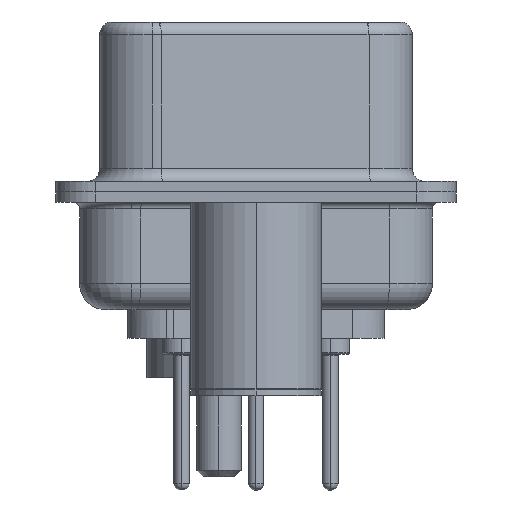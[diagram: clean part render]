
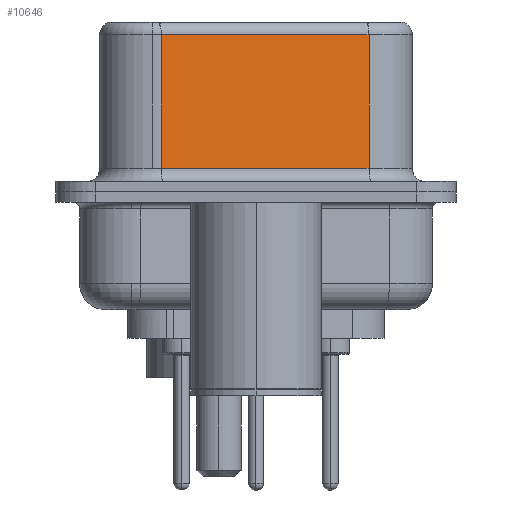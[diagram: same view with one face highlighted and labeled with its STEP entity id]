
A CAD part, left-side view. The second image highlights one B-rep face of the part: STEP entity #10646.
In plain terms, the highlighted planar face has unit normal (-0.985, -0.174, 0).
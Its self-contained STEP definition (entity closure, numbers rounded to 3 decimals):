
#1624 = CARTESIAN_POINT ( 'NONE',  ( 5.132, -4.322, 6.52 ) ) ;
#1778 = DIRECTION ( 'NONE',  ( 0., 0., -1. ) ) ;
#2152 = FACE_OUTER_BOUND ( 'NONE', #5448, .T. ) ;
#3857 = EDGE_CURVE ( 'NONE', #17078, #5729, #20822, .T. ) ;
#3877 = DIRECTION ( 'NONE',  ( -0.174, 0.985, 0. ) ) ;
#4196 = EDGE_CURVE ( 'NONE', #9244, #5729, #7252, .T. ) ;
#4510 = CARTESIAN_POINT ( 'NONE',  ( 5.132, -4.322, 6.52 ) ) ;
#4956 = VECTOR ( 'NONE', #6572, 1000. ) ;
#5448 = EDGE_LOOP ( 'NONE', ( #12501, #22151, #11166, #16965 ) ) ;
#5729 = VERTEX_POINT ( 'NONE', #16678 ) ;
#6572 = DIRECTION ( 'NONE',  ( 0., 0., -1. ) ) ;
#6870 = CARTESIAN_POINT ( 'NONE',  ( 5.132, -4.322, 6.02 ) ) ;
#7252 = LINE ( 'NONE', #4510, #12563 ) ;
#7342 = EDGE_CURVE ( 'NONE', #9244, #25363, #12393, .T. ) ;
#9244 = VERTEX_POINT ( 'NONE', #6870 ) ;
#10646 = ADVANCED_FACE ( 'NONE', ( #2152 ), #16500, .F. ) ;
#10993 = LINE ( 'NONE', #15505, #4956 ) ;
#11166 = ORIENTED_EDGE ( 'NONE', *, *, #28330, .T. ) ;
#11372 = DIRECTION ( 'NONE',  ( -0.174, 0.985, 0. ) ) ;
#12393 = LINE ( 'NONE', #13374, #17584 ) ;
#12501 = ORIENTED_EDGE ( 'NONE', *, *, #4196, .F. ) ;
#12563 = VECTOR ( 'NONE', #1778, 1000. ) ;
#13374 = CARTESIAN_POINT ( 'NONE',  ( 5.132, -4.322, 6.02 ) ) ;
#14955 = VECTOR ( 'NONE', #18409, 1000. ) ;
#15505 = CARTESIAN_POINT ( 'NONE',  ( 3.73, 3.628, 6.52 ) ) ;
#16500 = PLANE ( 'NONE',  #28735 ) ;
#16678 = CARTESIAN_POINT ( 'NONE',  ( 5.132, -4.322, 0.9 ) ) ;
#16965 = ORIENTED_EDGE ( 'NONE', *, *, #3857, .T. ) ;
#17078 = VERTEX_POINT ( 'NONE', #21581 ) ;
#17370 = DIRECTION ( 'NONE',  ( 0.985, 0.174, 0. ) ) ;
#17584 = VECTOR ( 'NONE', #11372, 1000. ) ;
#18409 = DIRECTION ( 'NONE',  ( 0.174, -0.985, 0. ) ) ;
#20822 = LINE ( 'NONE', #28739, #14955 ) ;
#21581 = CARTESIAN_POINT ( 'NONE',  ( 3.73, 3.628, 0.9 ) ) ;
#22151 = ORIENTED_EDGE ( 'NONE', *, *, #7342, .T. ) ;
#25363 = VERTEX_POINT ( 'NONE', #26192 ) ;
#26192 = CARTESIAN_POINT ( 'NONE',  ( 3.73, 3.628, 6.02 ) ) ;
#28330 = EDGE_CURVE ( 'NONE', #25363, #17078, #10993, .T. ) ;
#28735 = AXIS2_PLACEMENT_3D ( 'NONE', #1624, #17370, #3877 ) ;
#28739 = CARTESIAN_POINT ( 'NONE',  ( 5.132, -4.322, 0.9 ) ) ;
